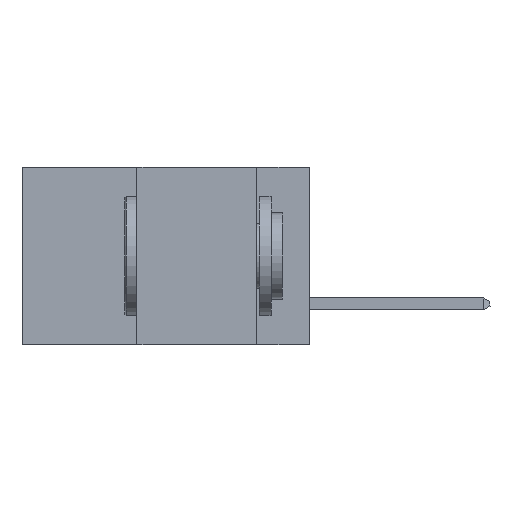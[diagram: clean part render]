
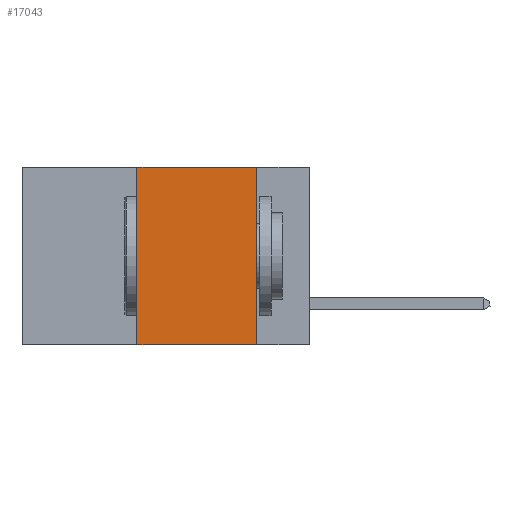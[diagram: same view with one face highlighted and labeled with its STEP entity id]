
A CAD part, left-side view. The second image highlights one B-rep face of the part: STEP entity #17043.
In plain terms, the highlighted planar face has unit normal (-1, 0, 0).
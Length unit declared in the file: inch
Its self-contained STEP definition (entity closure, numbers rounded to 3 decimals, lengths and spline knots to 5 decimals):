
#1698 = FACE_OUTER_BOUND ( 'NONE', #12215, .T. ) ;
#2308 = CARTESIAN_POINT ( 'NONE',  ( 0., 0.36, 0. ) ) ;
#2569 = EDGE_CURVE ( 'NONE', #16413, #11079, #18903, .T. ) ;
#2945 = DIRECTION ( 'NONE',  ( 0., -1., 0. ) ) ;
#3029 = VECTOR ( 'NONE', #17281, 39.37008 ) ;
#3111 = EDGE_CURVE ( 'NONE', #8404, #11079, #17811, .T. ) ;
#3906 = ORIENTED_EDGE ( 'NONE', *, *, #3111, .F. ) ;
#4027 = ORIENTED_EDGE ( 'NONE', *, *, #15478, .F. ) ;
#5083 = DIRECTION ( 'NONE',  ( 1., 0., 0. ) ) ;
#5371 = ORIENTED_EDGE ( 'NONE', *, *, #18387, .F. ) ;
#5827 = ORIENTED_EDGE ( 'NONE', *, *, #2569, .T. ) ;
#5946 = VECTOR ( 'NONE', #6298, 39.37008 ) ;
#6298 = DIRECTION ( 'NONE',  ( 0., 0., -1. ) ) ;
#6318 = CARTESIAN_POINT ( 'NONE',  ( 0., 0.11, 0. ) ) ;
#8404 = VERTEX_POINT ( 'NONE', #8596 ) ;
#8596 = CARTESIAN_POINT ( 'NONE',  ( 0., 0.11, 0. ) ) ;
#11079 = VERTEX_POINT ( 'NONE', #16114 ) ;
#11700 = VECTOR ( 'NONE', #2945, 39.37008 ) ;
#12044 = LINE ( 'NONE', #2308, #18749 ) ;
#12199 = CARTESIAN_POINT ( 'NONE',  ( 0., 0.6, 0. ) ) ;
#12215 = EDGE_LOOP ( 'NONE', ( #3906, #4027, #5371, #5827 ) ) ;
#12561 = CARTESIAN_POINT ( 'NONE',  ( 0., 0.36, -0.37 ) ) ;
#13566 = CARTESIAN_POINT ( 'NONE',  ( 0., 0.36, 0. ) ) ;
#14175 = PLANE ( 'NONE',  #14305 ) ;
#14305 = AXIS2_PLACEMENT_3D ( 'NONE', #18400, #5083, #15608 ) ;
#14439 = DIRECTION ( 'NONE',  ( 0., 0., 1. ) ) ;
#15478 = EDGE_CURVE ( 'NONE', #17963, #8404, #15536, .T. ) ;
#15536 = LINE ( 'NONE', #12199, #11700 ) ;
#15608 = DIRECTION ( 'NONE',  ( 0., 0., -1. ) ) ;
#16114 = CARTESIAN_POINT ( 'NONE',  ( 0., 0.11, -0.37 ) ) ;
#16413 = VERTEX_POINT ( 'NONE', #12561 ) ;
#17043 = ADVANCED_FACE ( 'NONE', ( #1698 ), #14175, .F. ) ;
#17281 = DIRECTION ( 'NONE',  ( 0., -1., 0. ) ) ;
#17588 = CARTESIAN_POINT ( 'NONE',  ( 0., 0.6, -0.37 ) ) ;
#17811 = LINE ( 'NONE', #6318, #5946 ) ;
#17963 = VERTEX_POINT ( 'NONE', #13566 ) ;
#18387 = EDGE_CURVE ( 'NONE', #16413, #17963, #12044, .T. ) ;
#18400 = CARTESIAN_POINT ( 'NONE',  ( 0., 0.6, 0. ) ) ;
#18749 = VECTOR ( 'NONE', #14439, 39.37008 ) ;
#18903 = LINE ( 'NONE', #17588, #3029 ) ;
